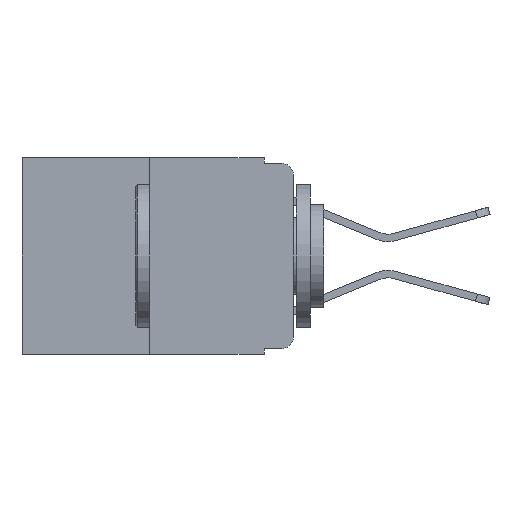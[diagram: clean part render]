
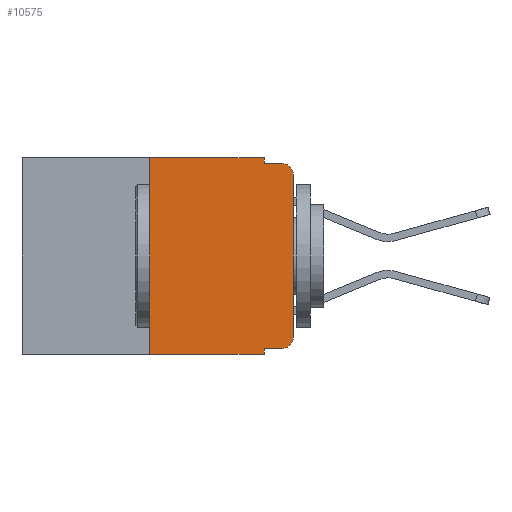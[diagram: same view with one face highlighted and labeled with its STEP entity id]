
A CAD part, left-side view. The second image highlights one B-rep face of the part: STEP entity #10575.
In plain terms, the highlighted planar face has unit normal (-1, 0, 0).
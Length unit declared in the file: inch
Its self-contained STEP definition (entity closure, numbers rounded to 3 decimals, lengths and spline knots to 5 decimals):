
#129 = DIRECTION ( 'NONE',  ( 1., 0., 0. ) ) ;
#177 = DIRECTION ( 'NONE',  ( -1., 0., 0. ) ) ;
#350 = VECTOR ( 'NONE', #9091, 39.37008 ) ;
#788 = LINE ( 'NONE', #3766, #350 ) ;
#864 = ORIENTED_EDGE ( 'NONE', *, *, #6699, .T. ) ;
#1570 = DIRECTION ( 'NONE',  ( 0., -1., 0. ) ) ;
#1682 = CARTESIAN_POINT ( 'NONE',  ( 0., 0.051, -0.01 ) ) ;
#2240 = CARTESIAN_POINT ( 'NONE',  ( 0., 0.25, 0. ) ) ;
#2787 = CARTESIAN_POINT ( 'NONE',  ( 0., 0.051, 0. ) ) ;
#2924 = CARTESIAN_POINT ( 'NONE',  ( 0., 0.473, 0. ) ) ;
#3033 = VERTEX_POINT ( 'NONE', #11102 ) ;
#3456 = AXIS2_PLACEMENT_3D ( 'NONE', #15320, #8062, #16503 ) ;
#3571 = VERTEX_POINT ( 'NONE', #15284 ) ;
#3766 = CARTESIAN_POINT ( 'NONE',  ( 0., 0.051, 0. ) ) ;
#3856 = LINE ( 'NONE', #7074, #6676 ) ;
#3931 = ORIENTED_EDGE ( 'NONE', *, *, #7090, .F. ) ;
#4169 = DIRECTION ( 'NONE',  ( 0., 0., -1. ) ) ;
#4420 = CARTESIAN_POINT ( 'NONE',  ( 0., 0.473, -0.343 ) ) ;
#4429 = VERTEX_POINT ( 'NONE', #7225 ) ;
#4475 = DIRECTION ( 'NONE',  ( 0., -1., 0. ) ) ;
#4569 = ORIENTED_EDGE ( 'NONE', *, *, #7278, .T. ) ;
#4570 = DIRECTION ( 'NONE',  ( 0., 0., 1. ) ) ;
#5243 = VERTEX_POINT ( 'NONE', #14343 ) ;
#5837 = CARTESIAN_POINT ( 'NONE',  ( 0., 0., -0.03 ) ) ;
#5980 = CARTESIAN_POINT ( 'NONE',  ( 0., 0., 0. ) ) ;
#6034 = LINE ( 'NONE', #11734, #8675 ) ;
#6239 = CIRCLE ( 'NONE', #8225, 0.02 ) ;
#6462 = EDGE_CURVE ( 'NONE', #3571, #15276, #15351, .T. ) ;
#6676 = VECTOR ( 'NONE', #8351, 39.37008 ) ;
#6699 = EDGE_CURVE ( 'NONE', #15276, #9968, #10031, .T. ) ;
#6782 = DIRECTION ( 'NONE',  ( 0., 0., 1. ) ) ;
#6829 = EDGE_CURVE ( 'NONE', #10680, #9968, #10206, .T. ) ;
#6830 = ORIENTED_EDGE ( 'NONE', *, *, #6829, .F. ) ;
#7074 = CARTESIAN_POINT ( 'NONE',  ( 0., 0.473, 0. ) ) ;
#7090 = EDGE_CURVE ( 'NONE', #13576, #10680, #788, .T. ) ;
#7091 = PLANE ( 'NONE',  #8149 ) ;
#7172 = EDGE_CURVE ( 'NONE', #3033, #16589, #6034, .T. ) ;
#7209 = EDGE_CURVE ( 'NONE', #10724, #4429, #8297, .T. ) ;
#7225 = CARTESIAN_POINT ( 'NONE',  ( 0., 0.051, -0.343 ) ) ;
#7235 = EDGE_CURVE ( 'NONE', #10724, #5243, #10762, .T. ) ;
#7256 = EDGE_CURVE ( 'NONE', #16589, #13576, #3856, .T. ) ;
#7278 = EDGE_CURVE ( 'NONE', #5243, #3571, #6239, .T. ) ;
#7507 = EDGE_CURVE ( 'NONE', #3033, #4429, #14372, .T. ) ;
#7509 = VECTOR ( 'NONE', #4475, 39.37008 ) ;
#8062 = DIRECTION ( 'NONE',  ( -1., 0., 0. ) ) ;
#8149 = AXIS2_PLACEMENT_3D ( 'NONE', #2924, #129, #9584 ) ;
#8225 = AXIS2_PLACEMENT_3D ( 'NONE', #8402, #177, #9626 ) ;
#8297 = LINE ( 'NONE', #2787, #14386 ) ;
#8301 = CARTESIAN_POINT ( 'NONE',  ( 0., 0.051, -0.333 ) ) ;
#8351 = DIRECTION ( 'NONE',  ( 0., -1., 0. ) ) ;
#8354 = EDGE_LOOP ( 'NONE', ( #15417, #864, #6830, #3931, #12964, #13077, #13296, #11978, #13252, #4569 ) ) ;
#8402 = CARTESIAN_POINT ( 'NONE',  ( 0., 0.02, -0.313 ) ) ;
#8667 = CARTESIAN_POINT ( 'NONE',  ( 0., 0.051, 0. ) ) ;
#8675 = VECTOR ( 'NONE', #6782, 39.37008 ) ;
#9091 = DIRECTION ( 'NONE',  ( 0., 0., -1. ) ) ;
#9195 = FACE_OUTER_BOUND ( 'NONE', #8354, .T. ) ;
#9520 = DIRECTION ( 'NONE',  ( 0., -1., 0. ) ) ;
#9584 = DIRECTION ( 'NONE',  ( 0., 0., -1. ) ) ;
#9626 = DIRECTION ( 'NONE',  ( 0., 0., -1. ) ) ;
#9740 = CARTESIAN_POINT ( 'NONE',  ( 0., 0.051, -0.333 ) ) ;
#9968 = VERTEX_POINT ( 'NONE', #14865 ) ;
#10031 = CIRCLE ( 'NONE', #3456, 0.02 ) ;
#10206 = LINE ( 'NONE', #15627, #16251 ) ;
#10371 = VECTOR ( 'NONE', #9520, 39.37008 ) ;
#10575 = ADVANCED_FACE ( 'NONE', ( #9195 ), #7091, .F. ) ;
#10680 = VERTEX_POINT ( 'NONE', #1682 ) ;
#10724 = VERTEX_POINT ( 'NONE', #9740 ) ;
#10762 = LINE ( 'NONE', #8301, #10371 ) ;
#11102 = CARTESIAN_POINT ( 'NONE',  ( 0., 0.25, -0.343 ) ) ;
#11732 = VECTOR ( 'NONE', #4570, 39.37008 ) ;
#11734 = CARTESIAN_POINT ( 'NONE',  ( 0., 0.25, 0. ) ) ;
#11978 = ORIENTED_EDGE ( 'NONE', *, *, #7209, .F. ) ;
#12964 = ORIENTED_EDGE ( 'NONE', *, *, #7256, .F. ) ;
#13077 = ORIENTED_EDGE ( 'NONE', *, *, #7172, .F. ) ;
#13252 = ORIENTED_EDGE ( 'NONE', *, *, #7235, .T. ) ;
#13296 = ORIENTED_EDGE ( 'NONE', *, *, #7507, .T. ) ;
#13576 = VERTEX_POINT ( 'NONE', #8667 ) ;
#14343 = CARTESIAN_POINT ( 'NONE',  ( 0., 0.02, -0.333 ) ) ;
#14372 = LINE ( 'NONE', #4420, #7509 ) ;
#14386 = VECTOR ( 'NONE', #4169, 39.37008 ) ;
#14865 = CARTESIAN_POINT ( 'NONE',  ( 0., 0.02, -0.01 ) ) ;
#15276 = VERTEX_POINT ( 'NONE', #5837 ) ;
#15284 = CARTESIAN_POINT ( 'NONE',  ( 0., 0., -0.313 ) ) ;
#15320 = CARTESIAN_POINT ( 'NONE',  ( 0., 0.02, -0.03 ) ) ;
#15351 = LINE ( 'NONE', #5980, #11732 ) ;
#15417 = ORIENTED_EDGE ( 'NONE', *, *, #6462, .T. ) ;
#15627 = CARTESIAN_POINT ( 'NONE',  ( 0., 0.051, -0.01 ) ) ;
#16251 = VECTOR ( 'NONE', #1570, 39.37008 ) ;
#16503 = DIRECTION ( 'NONE',  ( 0., 0., -1. ) ) ;
#16589 = VERTEX_POINT ( 'NONE', #2240 ) ;
